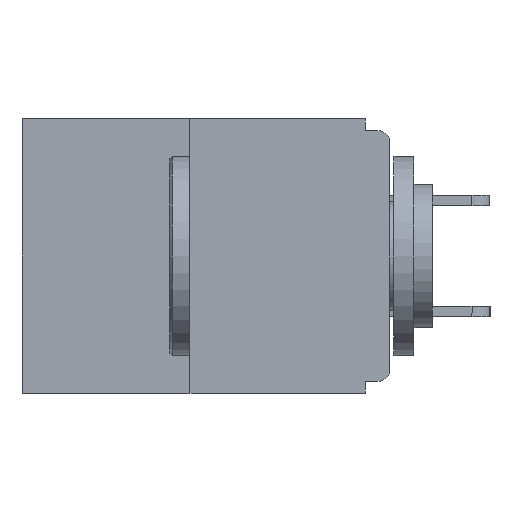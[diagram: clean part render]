
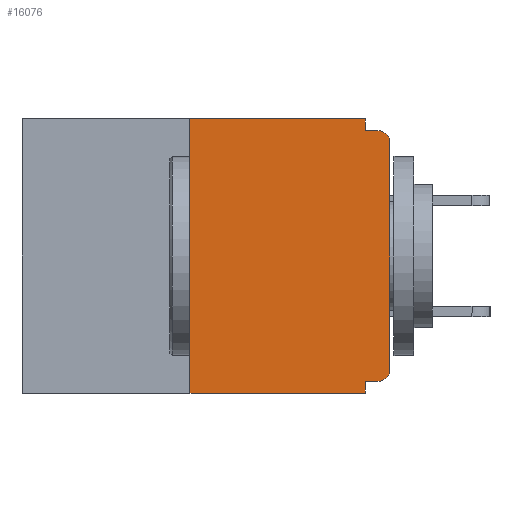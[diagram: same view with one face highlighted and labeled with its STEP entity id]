
A CAD part, left-side view. The second image highlights one B-rep face of the part: STEP entity #16076.
In plain terms, the highlighted planar face has unit normal (-1, 0, 0).
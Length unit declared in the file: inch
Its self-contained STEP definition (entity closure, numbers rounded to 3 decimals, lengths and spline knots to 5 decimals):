
#40 = VECTOR ( 'NONE', #17784, 39.37008 ) ;
#661 = CARTESIAN_POINT ( 'NONE',  ( 0., 0.015, -0.015 ) ) ;
#809 = ORIENTED_EDGE ( 'NONE', *, *, #3621, .T. ) ;
#1001 = DIRECTION ( 'NONE',  ( 0., 0., -1. ) ) ;
#1562 = CARTESIAN_POINT ( 'NONE',  ( 0., 0.46, -0.343 ) ) ;
#1750 = LINE ( 'NONE', #12440, #9980 ) ;
#1821 = DIRECTION ( 'NONE',  ( 0., 0., 1. ) ) ;
#2545 = VERTEX_POINT ( 'NONE', #2756 ) ;
#2756 = CARTESIAN_POINT ( 'NONE',  ( 0., 0.031, -0.343 ) ) ;
#3070 = LINE ( 'NONE', #5858, #3739 ) ;
#3376 = CARTESIAN_POINT ( 'NONE',  ( 0., 0.25, 0. ) ) ;
#3528 = DIRECTION ( 'NONE',  ( 0., 0., -1. ) ) ;
#3621 = EDGE_CURVE ( 'NONE', #23341, #22417, #18560, .T. ) ;
#3739 = VECTOR ( 'NONE', #1821, 39.37008 ) ;
#4040 = EDGE_CURVE ( 'NONE', #10067, #14845, #3070, .T. ) ;
#4523 = VECTOR ( 'NONE', #13539, 39.37008 ) ;
#5273 = AXIS2_PLACEMENT_3D ( 'NONE', #12452, #6193, #20386 ) ;
#5280 = EDGE_CURVE ( 'NONE', #10067, #2545, #13138, .T. ) ;
#5668 = VERTEX_POINT ( 'NONE', #17254 ) ;
#5858 = CARTESIAN_POINT ( 'NONE',  ( 0., 0.25, 0. ) ) ;
#5863 = DIRECTION ( 'NONE',  ( 0., -1., 0. ) ) ;
#5935 = VECTOR ( 'NONE', #21883, 39.37008 ) ;
#6193 = DIRECTION ( 'NONE',  ( -1., 0., 0. ) ) ;
#6839 = CIRCLE ( 'NONE', #5273, 0.015 ) ;
#7258 = EDGE_CURVE ( 'NONE', #16517, #2545, #15561, .T. ) ;
#7858 = CARTESIAN_POINT ( 'NONE',  ( 0., 0., -0.015 ) ) ;
#8348 = AXIS2_PLACEMENT_3D ( 'NONE', #12907, #15082, #1001 ) ;
#9297 = ORIENTED_EDGE ( 'NONE', *, *, #14605, .F. ) ;
#9421 = CARTESIAN_POINT ( 'NONE',  ( 0., 0.46, 0. ) ) ;
#9937 = CIRCLE ( 'NONE', #8348, 0.015 ) ;
#9980 = VECTOR ( 'NONE', #16662, 39.37008 ) ;
#10018 = ORIENTED_EDGE ( 'NONE', *, *, #5280, .T. ) ;
#10067 = VERTEX_POINT ( 'NONE', #12018 ) ;
#10327 = CARTESIAN_POINT ( 'NONE',  ( 0., 0.031, 0. ) ) ;
#10857 = FACE_OUTER_BOUND ( 'NONE', #22352, .T. ) ;
#10870 = ORIENTED_EDGE ( 'NONE', *, *, #14801, .F. ) ;
#11584 = ORIENTED_EDGE ( 'NONE', *, *, #4040, .F. ) ;
#11824 = EDGE_CURVE ( 'NONE', #5668, #23341, #6839, .T. ) ;
#12018 = CARTESIAN_POINT ( 'NONE',  ( 0., 0.25, -0.343 ) ) ;
#12440 = CARTESIAN_POINT ( 'NONE',  ( 0., 0., -0.328 ) ) ;
#12452 = CARTESIAN_POINT ( 'NONE',  ( 0., 0.015, -0.313 ) ) ;
#12483 = EDGE_CURVE ( 'NONE', #16643, #19142, #25512, .T. ) ;
#12648 = EDGE_CURVE ( 'NONE', #5668, #16517, #1750, .T. ) ;
#12695 = ORIENTED_EDGE ( 'NONE', *, *, #24301, .T. ) ;
#12907 = CARTESIAN_POINT ( 'NONE',  ( 0., 0.015, -0.03 ) ) ;
#12919 = VECTOR ( 'NONE', #15124, 39.37008 ) ;
#13138 = LINE ( 'NONE', #1562, #13767 ) ;
#13539 = DIRECTION ( 'NONE',  ( 0., -1., 0. ) ) ;
#13600 = DIRECTION ( 'NONE',  ( 1., 0., 0. ) ) ;
#13767 = VECTOR ( 'NONE', #5863, 39.37008 ) ;
#14157 = AXIS2_PLACEMENT_3D ( 'NONE', #9421, #13600, #3528 ) ;
#14319 = VECTOR ( 'NONE', #14393, 39.37008 ) ;
#14393 = DIRECTION ( 'NONE',  ( 0., 0., -1. ) ) ;
#14605 = EDGE_CURVE ( 'NONE', #20073, #16643, #17136, .T. ) ;
#14801 = EDGE_CURVE ( 'NONE', #14845, #20073, #23124, .T. ) ;
#14845 = VERTEX_POINT ( 'NONE', #3376 ) ;
#15082 = DIRECTION ( 'NONE',  ( -1., 0., 0. ) ) ;
#15124 = DIRECTION ( 'NONE',  ( 0., 0., 1. ) ) ;
#15217 = CARTESIAN_POINT ( 'NONE',  ( 0., 0., 0. ) ) ;
#15561 = LINE ( 'NONE', #16120, #40 ) ;
#15670 = CARTESIAN_POINT ( 'NONE',  ( 0., 0.031, -0.328 ) ) ;
#15856 = CARTESIAN_POINT ( 'NONE',  ( 0., 0., -0.313 ) ) ;
#16076 = ADVANCED_FACE ( 'NONE', ( #10857 ), #25709, .F. ) ;
#16120 = CARTESIAN_POINT ( 'NONE',  ( 0., 0.031, -0.343 ) ) ;
#16517 = VERTEX_POINT ( 'NONE', #15670 ) ;
#16643 = VERTEX_POINT ( 'NONE', #20065 ) ;
#16662 = DIRECTION ( 'NONE',  ( 0., 1., 0. ) ) ;
#17136 = LINE ( 'NONE', #10327, #14319 ) ;
#17254 = CARTESIAN_POINT ( 'NONE',  ( 0., 0.015, -0.328 ) ) ;
#17784 = DIRECTION ( 'NONE',  ( 0., 0., -1. ) ) ;
#18357 = ORIENTED_EDGE ( 'NONE', *, *, #7258, .F. ) ;
#18560 = LINE ( 'NONE', #15217, #12919 ) ;
#19069 = CARTESIAN_POINT ( 'NONE',  ( 0., 0., -0.03 ) ) ;
#19142 = VERTEX_POINT ( 'NONE', #661 ) ;
#19315 = ORIENTED_EDGE ( 'NONE', *, *, #12648, .F. ) ;
#19531 = ORIENTED_EDGE ( 'NONE', *, *, #11824, .T. ) ;
#20065 = CARTESIAN_POINT ( 'NONE',  ( 0., 0.031, -0.015 ) ) ;
#20073 = VERTEX_POINT ( 'NONE', #20572 ) ;
#20386 = DIRECTION ( 'NONE',  ( 0., 0., -1. ) ) ;
#20572 = CARTESIAN_POINT ( 'NONE',  ( 0., 0.031, 0. ) ) ;
#21883 = DIRECTION ( 'NONE',  ( 0., -1., 0. ) ) ;
#22352 = EDGE_LOOP ( 'NONE', ( #10870, #11584, #10018, #18357, #19315, #19531, #809, #12695, #26127, #9297 ) ) ;
#22417 = VERTEX_POINT ( 'NONE', #19069 ) ;
#23124 = LINE ( 'NONE', #23220, #4523 ) ;
#23220 = CARTESIAN_POINT ( 'NONE',  ( 0., 0.46, 0. ) ) ;
#23341 = VERTEX_POINT ( 'NONE', #15856 ) ;
#24301 = EDGE_CURVE ( 'NONE', #22417, #19142, #9937, .T. ) ;
#25512 = LINE ( 'NONE', #7858, #5935 ) ;
#25709 = PLANE ( 'NONE',  #14157 ) ;
#26127 = ORIENTED_EDGE ( 'NONE', *, *, #12483, .F. ) ;
